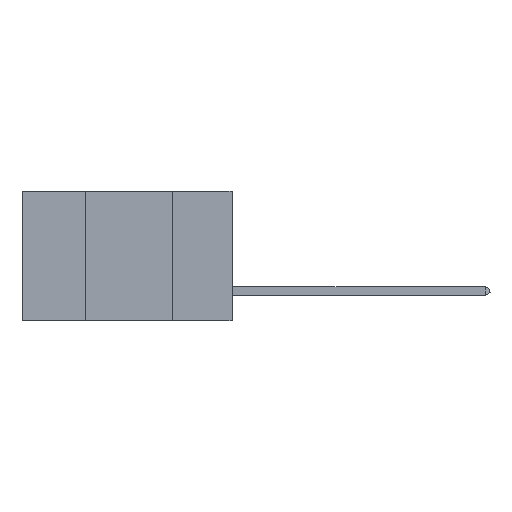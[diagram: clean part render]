
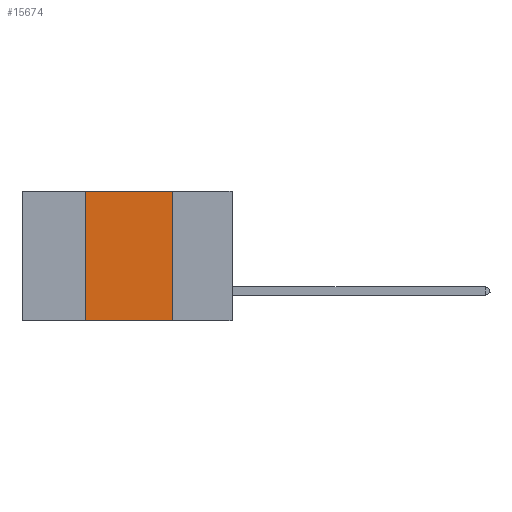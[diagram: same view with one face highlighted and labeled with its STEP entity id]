
A CAD part, left-side view. The second image highlights one B-rep face of the part: STEP entity #15674.
In plain terms, the highlighted planar face has unit normal (-1, 0, 0).
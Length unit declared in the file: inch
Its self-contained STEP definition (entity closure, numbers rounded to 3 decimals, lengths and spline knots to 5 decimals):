
#3072 = CARTESIAN_POINT ( 'NONE',  ( 0., 0.42, 0. ) ) ;
#3457 = EDGE_CURVE ( 'NONE', #18514, #23338, #10311, .T. ) ;
#4188 = DIRECTION ( 'NONE',  ( 0., 0., 1. ) ) ;
#4847 = CARTESIAN_POINT ( 'NONE',  ( 0., 0.17, -0.37 ) ) ;
#5452 = CARTESIAN_POINT ( 'NONE',  ( 0., 0.17, 0. ) ) ;
#6282 = CARTESIAN_POINT ( 'NONE',  ( 0., 0.42, 0. ) ) ;
#6786 = VECTOR ( 'NONE', #23223, 39.37008 ) ;
#7380 = DIRECTION ( 'NONE',  ( 0., 0., -1. ) ) ;
#8229 = EDGE_CURVE ( 'NONE', #24581, #16354, #12114, .T. ) ;
#8386 = DIRECTION ( 'NONE',  ( 0., 0., -1. ) ) ;
#8642 = EDGE_LOOP ( 'NONE', ( #24486, #15502, #9075, #14898 ) ) ;
#9075 = ORIENTED_EDGE ( 'NONE', *, *, #14283, .F. ) ;
#9782 = LINE ( 'NONE', #5452, #15168 ) ;
#10311 = LINE ( 'NONE', #15698, #13610 ) ;
#11153 = AXIS2_PLACEMENT_3D ( 'NONE', #21491, #11950, #8386 ) ;
#11709 = PLANE ( 'NONE',  #11153 ) ;
#11751 = VECTOR ( 'NONE', #4188, 39.37008 ) ;
#11950 = DIRECTION ( 'NONE',  ( 1., 0., 0. ) ) ;
#12114 = LINE ( 'NONE', #20588, #6786 ) ;
#13610 = VECTOR ( 'NONE', #21397, 39.37008 ) ;
#13776 = FACE_OUTER_BOUND ( 'NONE', #8642, .T. ) ;
#13817 = CARTESIAN_POINT ( 'NONE',  ( 0., 0.42, -0.37 ) ) ;
#14283 = EDGE_CURVE ( 'NONE', #24581, #18514, #18005, .T. ) ;
#14898 = ORIENTED_EDGE ( 'NONE', *, *, #8229, .T. ) ;
#15168 = VECTOR ( 'NONE', #7380, 39.37008 ) ;
#15502 = ORIENTED_EDGE ( 'NONE', *, *, #3457, .F. ) ;
#15674 = ADVANCED_FACE ( 'NONE', ( #13776 ), #11709, .F. ) ;
#15698 = CARTESIAN_POINT ( 'NONE',  ( 0., 0.6, 0. ) ) ;
#16354 = VERTEX_POINT ( 'NONE', #4847 ) ;
#17585 = EDGE_CURVE ( 'NONE', #23338, #16354, #9782, .T. ) ;
#18005 = LINE ( 'NONE', #6282, #11751 ) ;
#18514 = VERTEX_POINT ( 'NONE', #3072 ) ;
#19533 = CARTESIAN_POINT ( 'NONE',  ( 0., 0.17, 0. ) ) ;
#20588 = CARTESIAN_POINT ( 'NONE',  ( 0., 0.6, -0.37 ) ) ;
#21397 = DIRECTION ( 'NONE',  ( 0., -1., 0. ) ) ;
#21491 = CARTESIAN_POINT ( 'NONE',  ( 0., 0.6, 0. ) ) ;
#23223 = DIRECTION ( 'NONE',  ( 0., -1., 0. ) ) ;
#23338 = VERTEX_POINT ( 'NONE', #19533 ) ;
#24486 = ORIENTED_EDGE ( 'NONE', *, *, #17585, .F. ) ;
#24581 = VERTEX_POINT ( 'NONE', #13817 ) ;
